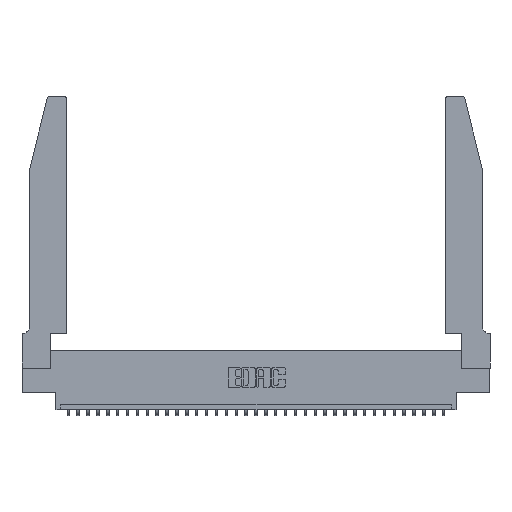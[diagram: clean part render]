
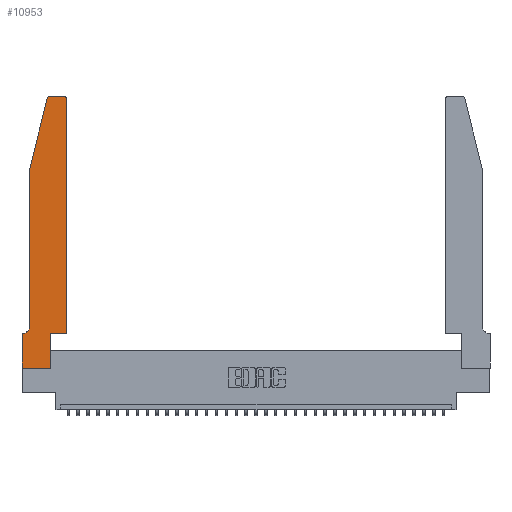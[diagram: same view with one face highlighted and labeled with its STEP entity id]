
A CAD part, top view. The second image highlights one B-rep face of the part: STEP entity #10953.
In plain terms, the highlighted planar face has unit normal (0, 0, 1).
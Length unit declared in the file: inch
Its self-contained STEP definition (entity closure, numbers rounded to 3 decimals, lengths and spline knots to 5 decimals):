
#107 = ORIENTED_EDGE ( 'NONE', *, *, #33597, .T. ) ;
#463 = VERTEX_POINT ( 'NONE', #14697 ) ;
#477 = DIRECTION ( 'NONE',  ( 1., 0., 0. ) ) ;
#1013 = LINE ( 'NONE', #13718, #23655 ) ;
#1042 = CARTESIAN_POINT ( 'NONE',  ( 0.25487, 2.72718, 0.37 ) ) ;
#1472 = LINE ( 'NONE', #9770, #5990 ) ;
#1560 = CARTESIAN_POINT ( 'NONE',  ( 0., 0.35, 0.37 ) ) ;
#2065 = DIRECTION ( 'NONE',  ( 0., 0., 1. ) ) ;
#2242 = VERTEX_POINT ( 'NONE', #10047 ) ;
#2418 = DIRECTION ( 'NONE',  ( 1., 0., 0. ) ) ;
#2881 = ORIENTED_EDGE ( 'NONE', *, *, #24309, .T. ) ;
#3818 = VERTEX_POINT ( 'NONE', #31692 ) ;
#4040 = ORIENTED_EDGE ( 'NONE', *, *, #29703, .T. ) ;
#4259 = CIRCLE ( 'NONE', #14871, 0.07 ) ;
#4528 = DIRECTION ( 'NONE',  ( -1., 0., 0. ) ) ;
#4743 = ORIENTED_EDGE ( 'NONE', *, *, #26633, .T. ) ;
#4910 = EDGE_CURVE ( 'NONE', #5981, #7314, #9282, .T. ) ;
#5981 = VERTEX_POINT ( 'NONE', #28450 ) ;
#5990 = VECTOR ( 'NONE', #9894, 39.37008 ) ;
#6516 = CARTESIAN_POINT ( 'NONE',  ( 0.4505, 0.35, 0.37 ) ) ;
#6688 = ORIENTED_EDGE ( 'NONE', *, *, #25010, .T. ) ;
#6721 = PLANE ( 'NONE',  #23792 ) ;
#6777 = CARTESIAN_POINT ( 'NONE',  ( 0.4505, 0.35, 0.37 ) ) ;
#6957 = CARTESIAN_POINT ( 'NONE',  ( 0.2605, 2.75, 0.37 ) ) ;
#7133 = VECTOR ( 'NONE', #4528, 39.37008 ) ;
#7150 = VECTOR ( 'NONE', #31951, 39.37008 ) ;
#7314 = VERTEX_POINT ( 'NONE', #28546 ) ;
#8564 = CIRCLE ( 'NONE', #32120, 0.03 ) ;
#9197 = LINE ( 'NONE', #23618, #7133 ) ;
#9282 = LINE ( 'NONE', #6957, #10942 ) ;
#9770 = CARTESIAN_POINT ( 'NONE',  ( 0.0755, 2., 0.37 ) ) ;
#9894 = DIRECTION ( 'NONE',  ( -0.239, -0.971, 0. ) ) ;
#10047 = CARTESIAN_POINT ( 'NONE',  ( 0., 0.35, 0.37 ) ) ;
#10054 = CARTESIAN_POINT ( 'NONE',  ( 0.4505, 0.35, 0.37 ) ) ;
#10095 = VECTOR ( 'NONE', #28316, 39.37008 ) ;
#10401 = CARTESIAN_POINT ( 'NONE',  ( 0.284, 2.72, 0.37 ) ) ;
#10942 = VECTOR ( 'NONE', #31199, 39.37008 ) ;
#10953 = ADVANCED_FACE ( 'NONE', ( #27007 ), #6721, .T. ) ;
#11110 = VECTOR ( 'NONE', #21336, 39.37008 ) ;
#11232 = VECTOR ( 'NONE', #2418, 39.37008 ) ;
#11277 = LINE ( 'NONE', #31609, #7150 ) ;
#12580 = ORIENTED_EDGE ( 'NONE', *, *, #24623, .T. ) ;
#12725 = EDGE_CURVE ( 'NONE', #14102, #5981, #8564, .T. ) ;
#13172 = DIRECTION ( 'NONE',  ( 1., 0., 0. ) ) ;
#13718 = CARTESIAN_POINT ( 'NONE',  ( 0., 0., 0.37 ) ) ;
#13745 = ORIENTED_EDGE ( 'NONE', *, *, #12725, .T. ) ;
#14102 = VERTEX_POINT ( 'NONE', #34677 ) ;
#14697 = CARTESIAN_POINT ( 'NONE',  ( 0.0755, 2., 0.37 ) ) ;
#14871 = AXIS2_PLACEMENT_3D ( 'NONE', #15206, #30588, #27992 ) ;
#15206 = CARTESIAN_POINT ( 'NONE',  ( 0.0055, 0.42, 0.37 ) ) ;
#15428 = DIRECTION ( 'NONE',  ( 1., 0., 0. ) ) ;
#15913 = EDGE_CURVE ( 'NONE', #29945, #2242, #9197, .T. ) ;
#16323 = VERTEX_POINT ( 'NONE', #31990 ) ;
#17229 = AXIS2_PLACEMENT_3D ( 'NONE', #10401, #2065, #31722 ) ;
#17702 = EDGE_LOOP ( 'NONE', ( #25753, #25302, #22168, #107, #22120, #18940, #12580, #4040, #6688, #4743, #2881, #13745 ) ) ;
#18940 = ORIENTED_EDGE ( 'NONE', *, *, #15913, .T. ) ;
#20268 = CARTESIAN_POINT ( 'NONE',  ( 0., 0., 0.37 ) ) ;
#21336 = DIRECTION ( 'NONE',  ( 0., -1., 0. ) ) ;
#21967 = EDGE_CURVE ( 'NONE', #31053, #463, #1472, .T. ) ;
#22120 = ORIENTED_EDGE ( 'NONE', *, *, #24167, .T. ) ;
#22168 = ORIENTED_EDGE ( 'NONE', *, *, #21967, .T. ) ;
#23010 = CARTESIAN_POINT ( 'NONE',  ( 0.0055, 0.35, 0.37 ) ) ;
#23618 = CARTESIAN_POINT ( 'NONE',  ( 0.0755, 0.35, 0.37 ) ) ;
#23655 = VECTOR ( 'NONE', #477, 39.37008 ) ;
#23792 = AXIS2_PLACEMENT_3D ( 'NONE', #1560, #31207, #13172 ) ;
#24167 = EDGE_CURVE ( 'NONE', #16323, #29945, #4259, .T. ) ;
#24309 = EDGE_CURVE ( 'NONE', #31361, #14102, #32731, .T. ) ;
#24623 = EDGE_CURVE ( 'NONE', #2242, #28705, #33364, .T. ) ;
#25010 = EDGE_CURVE ( 'NONE', #30113, #3818, #34460, .T. ) ;
#25302 = ORIENTED_EDGE ( 'NONE', *, *, #33606, .T. ) ;
#25753 = ORIENTED_EDGE ( 'NONE', *, *, #4910, .T. ) ;
#26633 = EDGE_CURVE ( 'NONE', #3818, #31361, #32643, .T. ) ;
#27007 = FACE_OUTER_BOUND ( 'NONE', #17702, .T. ) ;
#27992 = DIRECTION ( 'NONE',  ( -1., 0., 0. ) ) ;
#28316 = DIRECTION ( 'NONE',  ( 0., 1., 0. ) ) ;
#28450 = CARTESIAN_POINT ( 'NONE',  ( 0.4205, 2.75, 0.37 ) ) ;
#28546 = CARTESIAN_POINT ( 'NONE',  ( 0.284, 2.75, 0.37 ) ) ;
#28705 = VERTEX_POINT ( 'NONE', #20268 ) ;
#29703 = EDGE_CURVE ( 'NONE', #28705, #30113, #1013, .T. ) ;
#29945 = VERTEX_POINT ( 'NONE', #23010 ) ;
#30113 = VERTEX_POINT ( 'NONE', #34138 ) ;
#30588 = DIRECTION ( 'NONE',  ( 0., 0., -1. ) ) ;
#31053 = VERTEX_POINT ( 'NONE', #1042 ) ;
#31132 = DIRECTION ( 'NONE',  ( 0., 1., 0. ) ) ;
#31199 = DIRECTION ( 'NONE',  ( -1., 0., 0. ) ) ;
#31207 = DIRECTION ( 'NONE',  ( 0., 0., 1. ) ) ;
#31316 = DIRECTION ( 'NONE',  ( 0., 0., 1. ) ) ;
#31361 = VERTEX_POINT ( 'NONE', #6516 ) ;
#31609 = CARTESIAN_POINT ( 'NONE',  ( 0.0755, 2., 0.37 ) ) ;
#31651 = CARTESIAN_POINT ( 'NONE',  ( 0.4205, 2.72, 0.37 ) ) ;
#31692 = CARTESIAN_POINT ( 'NONE',  ( 0.2865, 0.35, 0.37 ) ) ;
#31722 = DIRECTION ( 'NONE',  ( 1., 0., 0. ) ) ;
#31951 = DIRECTION ( 'NONE',  ( 0., -1., 0. ) ) ;
#31990 = CARTESIAN_POINT ( 'NONE',  ( 0.0755, 0.42, 0.37 ) ) ;
#32047 = CARTESIAN_POINT ( 'NONE',  ( 0., 0., 0.37 ) ) ;
#32120 = AXIS2_PLACEMENT_3D ( 'NONE', #31651, #31316, #15428 ) ;
#32643 = LINE ( 'NONE', #10054, #11232 ) ;
#32685 = CIRCLE ( 'NONE', #17229, 0.03 ) ;
#32731 = LINE ( 'NONE', #6777, #10095 ) ;
#32768 = VECTOR ( 'NONE', #31132, 39.37008 ) ;
#33364 = LINE ( 'NONE', #32047, #11110 ) ;
#33597 = EDGE_CURVE ( 'NONE', #463, #16323, #11277, .T. ) ;
#33606 = EDGE_CURVE ( 'NONE', #7314, #31053, #32685, .T. ) ;
#34026 = CARTESIAN_POINT ( 'NONE',  ( 0.2865, 0.35, 0.37 ) ) ;
#34138 = CARTESIAN_POINT ( 'NONE',  ( 0.2865, 0., 0.37 ) ) ;
#34460 = LINE ( 'NONE', #34026, #32768 ) ;
#34677 = CARTESIAN_POINT ( 'NONE',  ( 0.4505, 2.72, 0.37 ) ) ;
